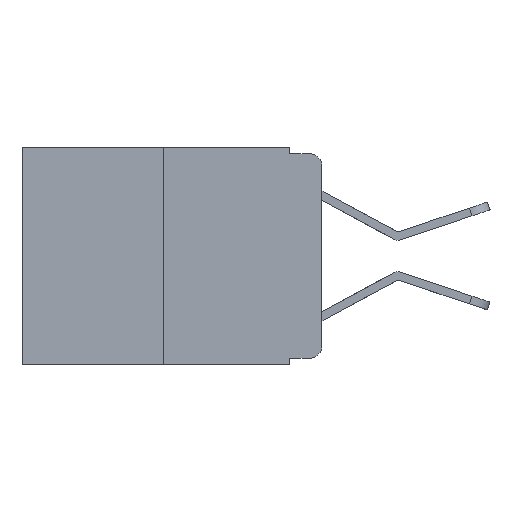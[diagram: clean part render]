
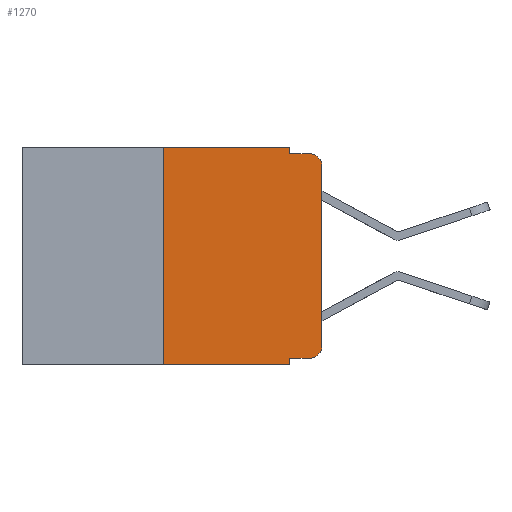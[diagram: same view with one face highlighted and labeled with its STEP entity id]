
A CAD part, left-side view. The second image highlights one B-rep face of the part: STEP entity #1270.
In plain terms, the highlighted planar face has unit normal (-1, 0, 0).
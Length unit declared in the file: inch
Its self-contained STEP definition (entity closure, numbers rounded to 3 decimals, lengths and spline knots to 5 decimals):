
#421 = EDGE_CURVE ( 'NONE', #5428, #1488, #12074, .T. ) ;
#443 = EDGE_CURVE ( 'NONE', #10073, #9223, #8578, .T. ) ;
#533 = CIRCLE ( 'NONE', #13551, 0.02 ) ;
#706 = ORIENTED_EDGE ( 'NONE', *, *, #1529, .T. ) ;
#711 = DIRECTION ( 'NONE',  ( 0., 0., -1. ) ) ;
#740 = ORIENTED_EDGE ( 'NONE', *, *, #11211, .F. ) ;
#838 = CARTESIAN_POINT ( 'NONE',  ( 0., 0.25, -0.343 ) ) ;
#983 = EDGE_CURVE ( 'NONE', #7957, #10180, #19580, .T. ) ;
#1270 = ADVANCED_FACE ( 'NONE', ( #10768 ), #11886, .F. ) ;
#1488 = VERTEX_POINT ( 'NONE', #14544 ) ;
#1529 = EDGE_CURVE ( 'NONE', #7957, #16891, #11251, .T. ) ;
#1843 = VECTOR ( 'NONE', #12899, 39.37008 ) ;
#1986 = EDGE_CURVE ( 'NONE', #10180, #12384, #12517, .T. ) ;
#2306 = CARTESIAN_POINT ( 'NONE',  ( 0., 0.02, -0.03 ) ) ;
#2325 = DIRECTION ( 'NONE',  ( 1., 0., 0. ) ) ;
#2364 = DIRECTION ( 'NONE',  ( 0., -1., 0. ) ) ;
#2370 = LINE ( 'NONE', #14114, #5604 ) ;
#2394 = CARTESIAN_POINT ( 'NONE',  ( 0., 0.473, 0. ) ) ;
#2453 = LINE ( 'NONE', #11098, #7427 ) ;
#2534 = CARTESIAN_POINT ( 'NONE',  ( 0., 0.051, -0.343 ) ) ;
#2573 = CARTESIAN_POINT ( 'NONE',  ( 0., 0., -0.313 ) ) ;
#2640 = DIRECTION ( 'NONE',  ( 0., 0., 1. ) ) ;
#3160 = ORIENTED_EDGE ( 'NONE', *, *, #983, .F. ) ;
#3218 = CARTESIAN_POINT ( 'NONE',  ( 0., 0.051, -0.333 ) ) ;
#3927 = CARTESIAN_POINT ( 'NONE',  ( 0., 0.473, -0.343 ) ) ;
#4029 = CARTESIAN_POINT ( 'NONE',  ( 0., 0.051, 0. ) ) ;
#4777 = VECTOR ( 'NONE', #13484, 39.37008 ) ;
#4783 = LINE ( 'NONE', #10149, #8988 ) ;
#5170 = DIRECTION ( 'NONE',  ( 0., 0., -1. ) ) ;
#5428 = VERTEX_POINT ( 'NONE', #3218 ) ;
#5604 = VECTOR ( 'NONE', #15774, 39.37008 ) ;
#5956 = VERTEX_POINT ( 'NONE', #2573 ) ;
#6181 = CARTESIAN_POINT ( 'NONE',  ( 0., 0.02, -0.01 ) ) ;
#6220 = DIRECTION ( 'NONE',  ( 0., 0., 1. ) ) ;
#6289 = VECTOR ( 'NONE', #2640, 39.37008 ) ;
#6333 = CARTESIAN_POINT ( 'NONE',  ( 0., 0.051, -0.01 ) ) ;
#7018 = VECTOR ( 'NONE', #2364, 39.37008 ) ;
#7321 = DIRECTION ( 'NONE',  ( -1., 0., 0. ) ) ;
#7427 = VECTOR ( 'NONE', #6220, 39.37008 ) ;
#7957 = VERTEX_POINT ( 'NONE', #838 ) ;
#8578 = LINE ( 'NONE', #6333, #1843 ) ;
#8731 = DIRECTION ( 'NONE',  ( 0., 0., -1. ) ) ;
#8988 = VECTOR ( 'NONE', #5170, 39.37008 ) ;
#9223 = VERTEX_POINT ( 'NONE', #6181 ) ;
#9331 = DIRECTION ( 'NONE',  ( 0., -1., 0. ) ) ;
#10073 = VERTEX_POINT ( 'NONE', #10239 ) ;
#10149 = CARTESIAN_POINT ( 'NONE',  ( 0., 0.051, 0. ) ) ;
#10180 = VERTEX_POINT ( 'NONE', #17056 ) ;
#10239 = CARTESIAN_POINT ( 'NONE',  ( 0., 0.051, -0.01 ) ) ;
#10387 = CARTESIAN_POINT ( 'NONE',  ( 0., 0., -0.03 ) ) ;
#10768 = FACE_OUTER_BOUND ( 'NONE', #11575, .T. ) ;
#11098 = CARTESIAN_POINT ( 'NONE',  ( 0., 0., 0. ) ) ;
#11104 = ORIENTED_EDGE ( 'NONE', *, *, #443, .F. ) ;
#11211 = EDGE_CURVE ( 'NONE', #12384, #10073, #4783, .T. ) ;
#11251 = LINE ( 'NONE', #3927, #4777 ) ;
#11575 = EDGE_LOOP ( 'NONE', ( #14874, #17418, #11104, #740, #19334, #3160, #706, #20161, #15288, #12616 ) ) ;
#11768 = EDGE_CURVE ( 'NONE', #12408, #9223, #533, .T. ) ;
#11886 = PLANE ( 'NONE',  #16053 ) ;
#12074 = LINE ( 'NONE', #14067, #16565 ) ;
#12384 = VERTEX_POINT ( 'NONE', #4029 ) ;
#12408 = VERTEX_POINT ( 'NONE', #10387 ) ;
#12517 = LINE ( 'NONE', #14082, #7018 ) ;
#12616 = ORIENTED_EDGE ( 'NONE', *, *, #15612, .T. ) ;
#12899 = DIRECTION ( 'NONE',  ( 0., -1., 0. ) ) ;
#13482 = DIRECTION ( 'NONE',  ( 0., 0., -1. ) ) ;
#13484 = DIRECTION ( 'NONE',  ( 0., -1., 0. ) ) ;
#13551 = AXIS2_PLACEMENT_3D ( 'NONE', #2306, #15265, #711 ) ;
#14067 = CARTESIAN_POINT ( 'NONE',  ( 0., 0.051, -0.333 ) ) ;
#14082 = CARTESIAN_POINT ( 'NONE',  ( 0., 0.473, 0. ) ) ;
#14114 = CARTESIAN_POINT ( 'NONE',  ( 0., 0.051, 0. ) ) ;
#14541 = EDGE_CURVE ( 'NONE', #5428, #16891, #2370, .T. ) ;
#14544 = CARTESIAN_POINT ( 'NONE',  ( 0., 0.02, -0.333 ) ) ;
#14874 = ORIENTED_EDGE ( 'NONE', *, *, #18242, .T. ) ;
#15265 = DIRECTION ( 'NONE',  ( -1., 0., 0. ) ) ;
#15288 = ORIENTED_EDGE ( 'NONE', *, *, #421, .T. ) ;
#15612 = EDGE_CURVE ( 'NONE', #1488, #5956, #17300, .T. ) ;
#15774 = DIRECTION ( 'NONE',  ( 0., 0., -1. ) ) ;
#16053 = AXIS2_PLACEMENT_3D ( 'NONE', #2394, #2325, #13482 ) ;
#16123 = AXIS2_PLACEMENT_3D ( 'NONE', #18255, #7321, #8731 ) ;
#16565 = VECTOR ( 'NONE', #9331, 39.37008 ) ;
#16891 = VERTEX_POINT ( 'NONE', #2534 ) ;
#17056 = CARTESIAN_POINT ( 'NONE',  ( 0., 0.25, 0. ) ) ;
#17300 = CIRCLE ( 'NONE', #16123, 0.02 ) ;
#17418 = ORIENTED_EDGE ( 'NONE', *, *, #11768, .T. ) ;
#18242 = EDGE_CURVE ( 'NONE', #5956, #12408, #2453, .T. ) ;
#18255 = CARTESIAN_POINT ( 'NONE',  ( 0., 0.02, -0.313 ) ) ;
#19334 = ORIENTED_EDGE ( 'NONE', *, *, #1986, .F. ) ;
#19580 = LINE ( 'NONE', #20182, #6289 ) ;
#20161 = ORIENTED_EDGE ( 'NONE', *, *, #14541, .F. ) ;
#20182 = CARTESIAN_POINT ( 'NONE',  ( 0., 0.25, 0. ) ) ;
